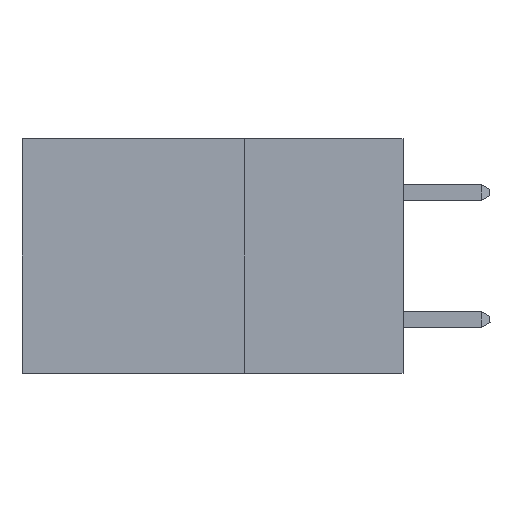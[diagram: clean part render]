
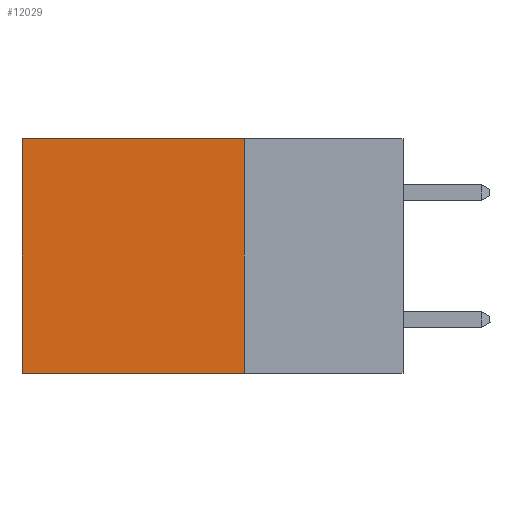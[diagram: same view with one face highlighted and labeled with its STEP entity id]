
A CAD part, left-side view. The second image highlights one B-rep face of the part: STEP entity #12029.
In plain terms, the highlighted planar face has unit normal (-1, 0, 0).
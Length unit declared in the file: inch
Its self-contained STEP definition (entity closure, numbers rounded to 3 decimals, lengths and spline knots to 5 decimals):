
#66 = LINE ( 'NONE', #8054, #4613 ) ;
#806 = CARTESIAN_POINT ( 'NONE',  ( 0.2875, 0.25, 0. ) ) ;
#3131 = PLANE ( 'NONE',  #14631 ) ;
#3750 = EDGE_CURVE ( 'NONE', #20334, #14385, #28074, .T. ) ;
#4613 = VECTOR ( 'NONE', #13136, 39.37008 ) ;
#5297 = VECTOR ( 'NONE', #18688, 39.37008 ) ;
#6266 = EDGE_CURVE ( 'NONE', #25474, #14385, #19291, .T. ) ;
#6521 = FACE_OUTER_BOUND ( 'NONE', #24463, .T. ) ;
#7648 = DIRECTION ( 'NONE',  ( 1., 0., 0. ) ) ;
#7773 = ORIENTED_EDGE ( 'NONE', *, *, #23585, .F. ) ;
#7855 = CARTESIAN_POINT ( 'NONE',  ( 0.2875, 0.25, 0. ) ) ;
#8054 = CARTESIAN_POINT ( 'NONE',  ( 0.2875, 0.25, 0. ) ) ;
#10042 = ORIENTED_EDGE ( 'NONE', *, *, #6266, .T. ) ;
#10091 = VERTEX_POINT ( 'NONE', #806 ) ;
#10157 = CARTESIAN_POINT ( 'NONE',  ( 0.2875, 0.6, 0. ) ) ;
#11707 = LINE ( 'NONE', #28268, #5297 ) ;
#12029 = ADVANCED_FACE ( 'NONE', ( #6521 ), #3131, .F. ) ;
#12726 = DIRECTION ( 'NONE',  ( 0., 0., -1. ) ) ;
#13136 = DIRECTION ( 'NONE',  ( 0., 0., -1. ) ) ;
#14385 = VERTEX_POINT ( 'NONE', #20543 ) ;
#14631 = AXIS2_PLACEMENT_3D ( 'NONE', #7855, #7648, #12726 ) ;
#15299 = VECTOR ( 'NONE', #16391, 39.37008 ) ;
#15614 = ORIENTED_EDGE ( 'NONE', *, *, #3750, .F. ) ;
#16088 = CARTESIAN_POINT ( 'NONE',  ( 0.2875, 0.25, -0.37 ) ) ;
#16391 = DIRECTION ( 'NONE',  ( 0., 1., 0. ) ) ;
#18688 = DIRECTION ( 'NONE',  ( 0., 1., 0. ) ) ;
#19291 = LINE ( 'NONE', #10157, #24160 ) ;
#19647 = DIRECTION ( 'NONE',  ( 0., 0., -1. ) ) ;
#20334 = VERTEX_POINT ( 'NONE', #22137 ) ;
#20543 = CARTESIAN_POINT ( 'NONE',  ( 0.2875, 0.6, -0.37 ) ) ;
#21068 = CARTESIAN_POINT ( 'NONE',  ( 0.2875, 0.6, 0. ) ) ;
#22137 = CARTESIAN_POINT ( 'NONE',  ( 0.2875, 0.25, -0.37 ) ) ;
#23585 = EDGE_CURVE ( 'NONE', #10091, #20334, #66, .T. ) ;
#24160 = VECTOR ( 'NONE', #19647, 39.37008 ) ;
#24463 = EDGE_LOOP ( 'NONE', ( #10042, #15614, #7773, #26978 ) ) ;
#25474 = VERTEX_POINT ( 'NONE', #21068 ) ;
#26978 = ORIENTED_EDGE ( 'NONE', *, *, #29098, .T. ) ;
#28074 = LINE ( 'NONE', #16088, #15299 ) ;
#28268 = CARTESIAN_POINT ( 'NONE',  ( 0.2875, 0.25, 0. ) ) ;
#29098 = EDGE_CURVE ( 'NONE', #10091, #25474, #11707, .T. ) ;
